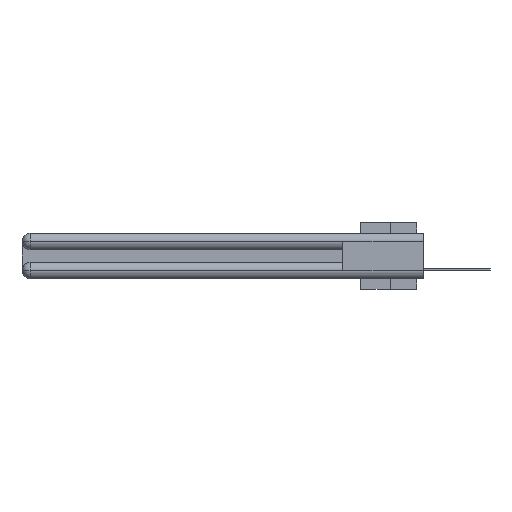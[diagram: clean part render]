
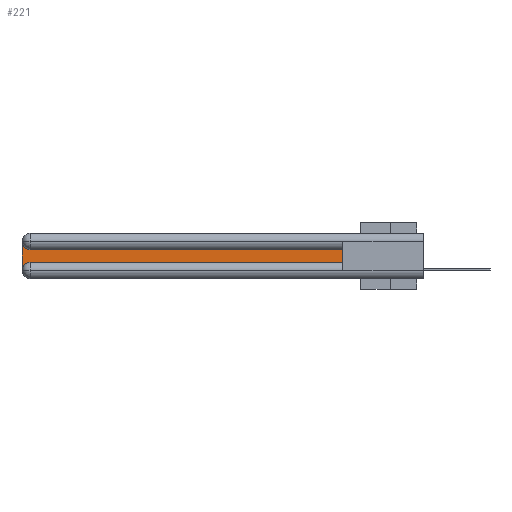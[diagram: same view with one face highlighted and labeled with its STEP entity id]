
A CAD part, left-side view. The second image highlights one B-rep face of the part: STEP entity #221.
In plain terms, the highlighted planar face has unit normal (-1, 0, 0).
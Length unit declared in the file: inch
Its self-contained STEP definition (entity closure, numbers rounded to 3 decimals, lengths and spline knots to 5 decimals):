
#10 = CARTESIAN_POINT ( 'NONE',  ( 0.075, 3., -0.2775 ) ) ;
#45 = DIRECTION ( 'NONE',  ( 1., 0., 0. ) ) ;
#221 = ADVANCED_FACE ( 'NONE', ( #32368 ), #13279, .F. ) ;
#709 = CARTESIAN_POINT ( 'NONE',  ( 0.075, 0.6, -0.1225 ) ) ;
#913 = AXIS2_PLACEMENT_3D ( 'NONE', #34750, #5436, #35663 ) ;
#1084 = VERTEX_POINT ( 'NONE', #30451 ) ;
#1930 = ORIENTED_EDGE ( 'NONE', *, *, #17223, .T. ) ;
#2101 = VERTEX_POINT ( 'NONE', #31179 ) ;
#2573 = CARTESIAN_POINT ( 'NONE',  ( 0.075, 0.6, -0.2175 ) ) ;
#3669 = EDGE_CURVE ( 'NONE', #1084, #5671, #37759, .T. ) ;
#3932 = EDGE_CURVE ( 'NONE', #2101, #28453, #19355, .T. ) ;
#4177 = AXIS2_PLACEMENT_3D ( 'NONE', #10602, #45, #9186 ) ;
#4412 = LINE ( 'NONE', #31839, #30336 ) ;
#4855 = AXIS2_PLACEMENT_3D ( 'NONE', #25616, #37789, #10501 ) ;
#5436 = DIRECTION ( 'NONE',  ( 1., 0., 0. ) ) ;
#5671 = VERTEX_POINT ( 'NONE', #10 ) ;
#6179 = CIRCLE ( 'NONE', #4177, 0.06 ) ;
#6462 = ORIENTED_EDGE ( 'NONE', *, *, #3932, .T. ) ;
#9186 = DIRECTION ( 'NONE',  ( 0., 0., -1. ) ) ;
#10161 = ORIENTED_EDGE ( 'NONE', *, *, #3669, .T. ) ;
#10475 = DIRECTION ( 'NONE',  ( 0., 0., -1. ) ) ;
#10501 = DIRECTION ( 'NONE',  ( 0., 0., -1. ) ) ;
#10602 = CARTESIAN_POINT ( 'NONE',  ( 0.075, 2.94, -0.2775 ) ) ;
#13279 = PLANE ( 'NONE',  #4855 ) ;
#13928 = DIRECTION ( 'NONE',  ( 0., 0., 1. ) ) ;
#14226 = CIRCLE ( 'NONE', #913, 0.06 ) ;
#15355 = VERTEX_POINT ( 'NONE', #2573 ) ;
#15465 = ORIENTED_EDGE ( 'NONE', *, *, #37780, .T. ) ;
#17159 = LINE ( 'NONE', #29704, #36249 ) ;
#17201 = CARTESIAN_POINT ( 'NONE',  ( 0.075, 3., -0.2175 ) ) ;
#17223 = EDGE_CURVE ( 'NONE', #28453, #1084, #14226, .T. ) ;
#18501 = VECTOR ( 'NONE', #37518, 39.37008 ) ;
#19355 = LINE ( 'NONE', #709, #18501 ) ;
#21719 = EDGE_LOOP ( 'NONE', ( #6462, #1930, #10161, #23962, #23258, #15465 ) ) ;
#23258 = ORIENTED_EDGE ( 'NONE', *, *, #27910, .T. ) ;
#23336 = DIRECTION ( 'NONE',  ( 0., -1., 0. ) ) ;
#23962 = ORIENTED_EDGE ( 'NONE', *, *, #36125, .T. ) ;
#25616 = CARTESIAN_POINT ( 'NONE',  ( 0.075, 3., -0.1225 ) ) ;
#27910 = EDGE_CURVE ( 'NONE', #29827, #15355, #17159, .T. ) ;
#28453 = VERTEX_POINT ( 'NONE', #28872 ) ;
#28872 = CARTESIAN_POINT ( 'NONE',  ( 0.075, 2.94, -0.1225 ) ) ;
#29704 = CARTESIAN_POINT ( 'NONE',  ( 0.075, 0.6, -0.2175 ) ) ;
#29827 = VERTEX_POINT ( 'NONE', #36428 ) ;
#30336 = VECTOR ( 'NONE', #13928, 39.37008 ) ;
#30451 = CARTESIAN_POINT ( 'NONE',  ( 0.075, 3., -0.0625 ) ) ;
#31179 = CARTESIAN_POINT ( 'NONE',  ( 0.075, 0.6, -0.1225 ) ) ;
#31839 = CARTESIAN_POINT ( 'NONE',  ( 0.075, 0.6, -0.2175 ) ) ;
#32368 = FACE_OUTER_BOUND ( 'NONE', #21719, .T. ) ;
#34750 = CARTESIAN_POINT ( 'NONE',  ( 0.075, 2.94, -0.0625 ) ) ;
#35663 = DIRECTION ( 'NONE',  ( 0., 0., -1. ) ) ;
#36125 = EDGE_CURVE ( 'NONE', #5671, #29827, #6179, .T. ) ;
#36249 = VECTOR ( 'NONE', #23336, 39.37008 ) ;
#36428 = CARTESIAN_POINT ( 'NONE',  ( 0.075, 2.94, -0.2175 ) ) ;
#36924 = VECTOR ( 'NONE', #10475, 39.37008 ) ;
#37518 = DIRECTION ( 'NONE',  ( 0., 1., 0. ) ) ;
#37759 = LINE ( 'NONE', #17201, #36924 ) ;
#37780 = EDGE_CURVE ( 'NONE', #15355, #2101, #4412, .T. ) ;
#37789 = DIRECTION ( 'NONE',  ( 1., 0., 0. ) ) ;
